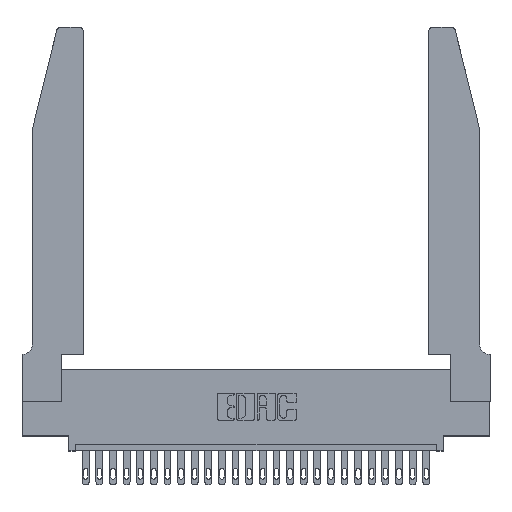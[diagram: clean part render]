
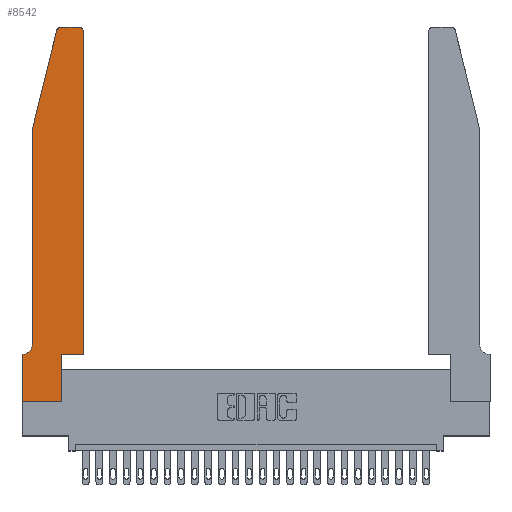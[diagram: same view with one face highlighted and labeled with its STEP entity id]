
A CAD part, top view. The second image highlights one B-rep face of the part: STEP entity #8542.
In plain terms, the highlighted planar face has unit normal (0, 0, 1).
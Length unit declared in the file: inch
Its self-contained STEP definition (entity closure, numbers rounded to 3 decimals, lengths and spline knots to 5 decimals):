
#212 = PLANE ( 'NONE',  #17970 ) ;
#1066 = LINE ( 'NONE', #25618, #2032 ) ;
#1330 = CARTESIAN_POINT ( 'NONE',  ( 0.4205, 2.72, 0.37 ) ) ;
#2032 = VECTOR ( 'NONE', #25529, 39.37008 ) ;
#2200 = EDGE_CURVE ( 'NONE', #3531, #4404, #13843, .T. ) ;
#2268 = VERTEX_POINT ( 'NONE', #10874 ) ;
#3018 = AXIS2_PLACEMENT_3D ( 'NONE', #5846, #7919, #26466 ) ;
#3531 = VERTEX_POINT ( 'NONE', #13949 ) ;
#3923 = VECTOR ( 'NONE', #18199, 39.37008 ) ;
#3939 = ORIENTED_EDGE ( 'NONE', *, *, #18038, .T. ) ;
#4144 = AXIS2_PLACEMENT_3D ( 'NONE', #1330, #15642, #19761 ) ;
#4404 = VERTEX_POINT ( 'NONE', #15790 ) ;
#4799 = VERTEX_POINT ( 'NONE', #13260 ) ;
#4956 = EDGE_CURVE ( 'NONE', #2268, #20561, #12074, .T. ) ;
#5846 = CARTESIAN_POINT ( 'NONE',  ( 0.284, 2.72, 0.37 ) ) ;
#6021 = CARTESIAN_POINT ( 'NONE',  ( 0.0755, 0.35, 0.37 ) ) ;
#6083 = DIRECTION ( 'NONE',  ( -0.239, -0.971, 0. ) ) ;
#6301 = DIRECTION ( 'NONE',  ( 0., 0., -1. ) ) ;
#6515 = VECTOR ( 'NONE', #8282, 39.37008 ) ;
#6714 = EDGE_CURVE ( 'NONE', #15179, #9519, #19595, .T. ) ;
#7197 = CARTESIAN_POINT ( 'NONE',  ( 0.0755, 2., 0.37 ) ) ;
#7880 = LINE ( 'NONE', #10127, #25219 ) ;
#7919 = DIRECTION ( 'NONE',  ( 0., 0., 1. ) ) ;
#8048 = LINE ( 'NONE', #9944, #24761 ) ;
#8280 = VERTEX_POINT ( 'NONE', #7197 ) ;
#8282 = DIRECTION ( 'NONE',  ( -1., 0., 0. ) ) ;
#8452 = DIRECTION ( 'NONE',  ( 0., 0., 1. ) ) ;
#8467 = CARTESIAN_POINT ( 'NONE',  ( 0.25487, 2.72718, 0.37 ) ) ;
#8542 = ADVANCED_FACE ( 'NONE', ( #9913 ), #212, .T. ) ;
#9122 = CARTESIAN_POINT ( 'NONE',  ( 0.2605, 2.75, 0.37 ) ) ;
#9519 = VERTEX_POINT ( 'NONE', #11381 ) ;
#9644 = VECTOR ( 'NONE', #23456, 39.37008 ) ;
#9823 = ORIENTED_EDGE ( 'NONE', *, *, #16228, .T. ) ;
#9913 = FACE_OUTER_BOUND ( 'NONE', #10708, .T. ) ;
#9944 = CARTESIAN_POINT ( 'NONE',  ( 0.4505, 0.35, 0.37 ) ) ;
#10045 = DIRECTION ( 'NONE',  ( 0., 1., 0. ) ) ;
#10127 = CARTESIAN_POINT ( 'NONE',  ( 0.0755, 2., 0.37 ) ) ;
#10254 = CARTESIAN_POINT ( 'NONE',  ( 0.0055, 0.42, 0.37 ) ) ;
#10350 = EDGE_CURVE ( 'NONE', #21053, #14558, #21997, .T. ) ;
#10390 = EDGE_CURVE ( 'NONE', #20993, #8280, #7880, .T. ) ;
#10694 = LINE ( 'NONE', #15893, #17442 ) ;
#10708 = EDGE_LOOP ( 'NONE', ( #12126, #9823, #11577, #18020, #14820, #3939, #11509, #14031, #12060, #10822, #17736, #25113 ) ) ;
#10822 = ORIENTED_EDGE ( 'NONE', *, *, #13758, .T. ) ;
#10874 = CARTESIAN_POINT ( 'NONE',  ( 0., 0.35, 0.37 ) ) ;
#11381 = CARTESIAN_POINT ( 'NONE',  ( 0.284, 2.75, 0.37 ) ) ;
#11509 = ORIENTED_EDGE ( 'NONE', *, *, #4956, .T. ) ;
#11577 = ORIENTED_EDGE ( 'NONE', *, *, #10390, .T. ) ;
#11784 = DIRECTION ( 'NONE',  ( 0., -1., 0. ) ) ;
#11929 = CARTESIAN_POINT ( 'NONE',  ( 0.2865, 0.35, 0.37 ) ) ;
#12060 = ORIENTED_EDGE ( 'NONE', *, *, #10350, .T. ) ;
#12074 = LINE ( 'NONE', #26332, #14000 ) ;
#12126 = ORIENTED_EDGE ( 'NONE', *, *, #6714, .T. ) ;
#12234 = LINE ( 'NONE', #20268, #3923 ) ;
#12574 = VERTEX_POINT ( 'NONE', #21060 ) ;
#13053 = CARTESIAN_POINT ( 'NONE',  ( 0.2865, 0.35, 0.37 ) ) ;
#13260 = CARTESIAN_POINT ( 'NONE',  ( 0.4505, 2.72, 0.37 ) ) ;
#13758 = EDGE_CURVE ( 'NONE', #14558, #12574, #12234, .T. ) ;
#13843 = CIRCLE ( 'NONE', #21658, 0.07 ) ;
#13949 = CARTESIAN_POINT ( 'NONE',  ( 0.0755, 0.42, 0.37 ) ) ;
#14000 = VECTOR ( 'NONE', #16193, 39.37008 ) ;
#14031 = ORIENTED_EDGE ( 'NONE', *, *, #24696, .T. ) ;
#14099 = EDGE_CURVE ( 'NONE', #12574, #4799, #8048, .T. ) ;
#14558 = VERTEX_POINT ( 'NONE', #13053 ) ;
#14820 = ORIENTED_EDGE ( 'NONE', *, *, #2200, .T. ) ;
#15179 = VERTEX_POINT ( 'NONE', #22907 ) ;
#15642 = DIRECTION ( 'NONE',  ( 0., 0., 1. ) ) ;
#15790 = CARTESIAN_POINT ( 'NONE',  ( 0.0055, 0.35, 0.37 ) ) ;
#15893 = CARTESIAN_POINT ( 'NONE',  ( 0.0755, 2., 0.37 ) ) ;
#16193 = DIRECTION ( 'NONE',  ( 0., -1., 0. ) ) ;
#16228 = EDGE_CURVE ( 'NONE', #9519, #20993, #23645, .T. ) ;
#16499 = DIRECTION ( 'NONE',  ( 1., 0., 0. ) ) ;
#16530 = VECTOR ( 'NONE', #10045, 39.37008 ) ;
#17442 = VECTOR ( 'NONE', #11784, 39.37008 ) ;
#17736 = ORIENTED_EDGE ( 'NONE', *, *, #14099, .T. ) ;
#17967 = EDGE_CURVE ( 'NONE', #8280, #3531, #10694, .T. ) ;
#17970 = AXIS2_PLACEMENT_3D ( 'NONE', #22511, #8452, #16499 ) ;
#18020 = ORIENTED_EDGE ( 'NONE', *, *, #17967, .T. ) ;
#18038 = EDGE_CURVE ( 'NONE', #4404, #2268, #25494, .T. ) ;
#18199 = DIRECTION ( 'NONE',  ( 1., 0., 0. ) ) ;
#19595 = LINE ( 'NONE', #9122, #9644 ) ;
#19761 = DIRECTION ( 'NONE',  ( 1., 0., 0. ) ) ;
#19986 = DIRECTION ( 'NONE',  ( 0., 1., 0. ) ) ;
#20268 = CARTESIAN_POINT ( 'NONE',  ( 0.4505, 0.35, 0.37 ) ) ;
#20561 = VERTEX_POINT ( 'NONE', #25186 ) ;
#20578 = DIRECTION ( 'NONE',  ( -1., 0., 0. ) ) ;
#20675 = CARTESIAN_POINT ( 'NONE',  ( 0.2865, 0., 0.37 ) ) ;
#20993 = VERTEX_POINT ( 'NONE', #8467 ) ;
#21053 = VERTEX_POINT ( 'NONE', #20675 ) ;
#21060 = CARTESIAN_POINT ( 'NONE',  ( 0.4505, 0.35, 0.37 ) ) ;
#21658 = AXIS2_PLACEMENT_3D ( 'NONE', #10254, #6301, #20578 ) ;
#21997 = LINE ( 'NONE', #11929, #16530 ) ;
#22511 = CARTESIAN_POINT ( 'NONE',  ( 0., 0.35, 0.37 ) ) ;
#22907 = CARTESIAN_POINT ( 'NONE',  ( 0.4205, 2.75, 0.37 ) ) ;
#23456 = DIRECTION ( 'NONE',  ( -1., 0., 0. ) ) ;
#23645 = CIRCLE ( 'NONE', #3018, 0.03 ) ;
#24696 = EDGE_CURVE ( 'NONE', #20561, #21053, #1066, .T. ) ;
#24761 = VECTOR ( 'NONE', #19986, 39.37008 ) ;
#25113 = ORIENTED_EDGE ( 'NONE', *, *, #26291, .T. ) ;
#25186 = CARTESIAN_POINT ( 'NONE',  ( 0., 0., 0.37 ) ) ;
#25219 = VECTOR ( 'NONE', #6083, 39.37008 ) ;
#25494 = LINE ( 'NONE', #6021, #6515 ) ;
#25529 = DIRECTION ( 'NONE',  ( 1., 0., 0. ) ) ;
#25618 = CARTESIAN_POINT ( 'NONE',  ( 0., 0., 0.37 ) ) ;
#25893 = CIRCLE ( 'NONE', #4144, 0.03 ) ;
#26291 = EDGE_CURVE ( 'NONE', #4799, #15179, #25893, .T. ) ;
#26332 = CARTESIAN_POINT ( 'NONE',  ( 0., 0., 0.37 ) ) ;
#26466 = DIRECTION ( 'NONE',  ( 1., 0., 0. ) ) ;
